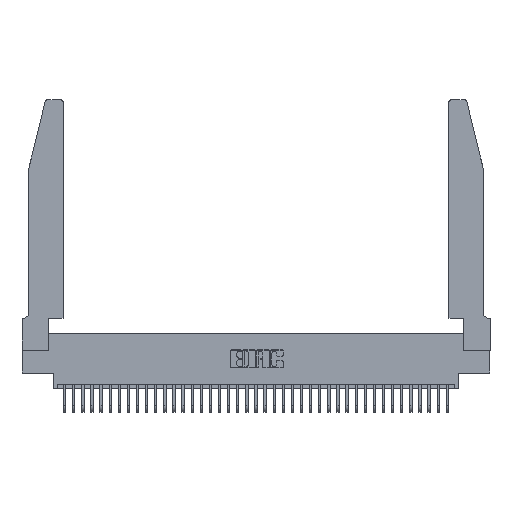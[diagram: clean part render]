
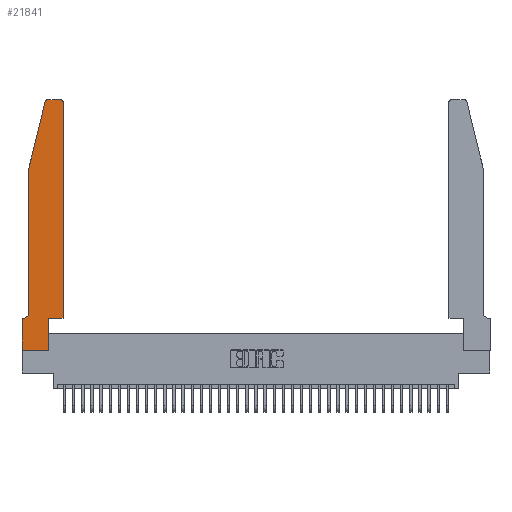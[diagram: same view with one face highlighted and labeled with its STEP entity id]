
A CAD part, top view. The second image highlights one B-rep face of the part: STEP entity #21841.
In plain terms, the highlighted planar face has unit normal (0, 0, 1).
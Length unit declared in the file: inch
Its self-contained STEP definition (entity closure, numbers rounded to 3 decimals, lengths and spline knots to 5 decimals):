
#62 = EDGE_CURVE ( 'NONE', #2987, #4222, #34412, .T. ) ;
#102 = VECTOR ( 'NONE', #3313, 39.37008 ) ;
#933 = VERTEX_POINT ( 'NONE', #10836 ) ;
#972 = CARTESIAN_POINT ( 'NONE',  ( 0., 0., 0.37 ) ) ;
#1541 = EDGE_CURVE ( 'NONE', #31274, #18560, #9662, .T. ) ;
#2202 = ORIENTED_EDGE ( 'NONE', *, *, #29389, .T. ) ;
#2729 = CARTESIAN_POINT ( 'NONE',  ( 0.4505, 0.35, 0.37 ) ) ;
#2750 = VERTEX_POINT ( 'NONE', #28711 ) ;
#2987 = VERTEX_POINT ( 'NONE', #12644 ) ;
#3313 = DIRECTION ( 'NONE',  ( 1., 0., 0. ) ) ;
#3594 = ORIENTED_EDGE ( 'NONE', *, *, #25880, .T. ) ;
#3938 = EDGE_CURVE ( 'NONE', #933, #15047, #12264, .T. ) ;
#4116 = ORIENTED_EDGE ( 'NONE', *, *, #21458, .T. ) ;
#4222 = VERTEX_POINT ( 'NONE', #32093 ) ;
#4388 = DIRECTION ( 'NONE',  ( 0., 0., -1. ) ) ;
#6137 = LINE ( 'NONE', #28819, #35675 ) ;
#6713 = DIRECTION ( 'NONE',  ( 0., 1., 0. ) ) ;
#6797 = CARTESIAN_POINT ( 'NONE',  ( 0.0755, 0.42, 0.37 ) ) ;
#7261 = AXIS2_PLACEMENT_3D ( 'NONE', #25074, #7840, #27955 ) ;
#7658 = ORIENTED_EDGE ( 'NONE', *, *, #17595, .T. ) ;
#7794 = CIRCLE ( 'NONE', #7261, 0.03 ) ;
#7840 = DIRECTION ( 'NONE',  ( 0., 0., 1. ) ) ;
#8736 = EDGE_LOOP ( 'NONE', ( #4116, #7658, #26403, #24208, #19255, #18488, #2202, #29838, #17821, #16942, #3594, #21818 ) ) ;
#9355 = LINE ( 'NONE', #22764, #23757 ) ;
#9662 = LINE ( 'NONE', #2729, #33421 ) ;
#10003 = DIRECTION ( 'NONE',  ( 0., 0., 1. ) ) ;
#10808 = DIRECTION ( 'NONE',  ( -1., 0., 0. ) ) ;
#10836 = CARTESIAN_POINT ( 'NONE',  ( 0.0055, 0.35, 0.37 ) ) ;
#11283 = VERTEX_POINT ( 'NONE', #972 ) ;
#11332 = CARTESIAN_POINT ( 'NONE',  ( 0.25487, 2.72718, 0.37 ) ) ;
#11401 = AXIS2_PLACEMENT_3D ( 'NONE', #27223, #10003, #30077 ) ;
#12264 = LINE ( 'NONE', #36436, #18083 ) ;
#12644 = CARTESIAN_POINT ( 'NONE',  ( 0.4505, 2.72, 0.37 ) ) ;
#12943 = LINE ( 'NONE', #35268, #28207 ) ;
#13743 = PLANE ( 'NONE',  #33267 ) ;
#13778 = CARTESIAN_POINT ( 'NONE',  ( 0.2865, 0., 0.37 ) ) ;
#14523 = DIRECTION ( 'NONE',  ( -1., 0., 0. ) ) ;
#15047 = VERTEX_POINT ( 'NONE', #26535 ) ;
#16609 = DIRECTION ( 'NONE',  ( 1., 0., 0. ) ) ;
#16890 = CARTESIAN_POINT ( 'NONE',  ( 0.0755, 2., 0.37 ) ) ;
#16942 = ORIENTED_EDGE ( 'NONE', *, *, #1541, .T. ) ;
#17369 = EDGE_CURVE ( 'NONE', #35594, #31274, #31142, .T. ) ;
#17595 = EDGE_CURVE ( 'NONE', #28158, #18311, #7794, .T. ) ;
#17821 = ORIENTED_EDGE ( 'NONE', *, *, #17369, .T. ) ;
#17947 = CARTESIAN_POINT ( 'NONE',  ( 0.4505, 0.35, 0.37 ) ) ;
#18083 = VECTOR ( 'NONE', #10808, 39.37008 ) ;
#18183 = DIRECTION ( 'NONE',  ( -0.239, -0.971, 0. ) ) ;
#18311 = VERTEX_POINT ( 'NONE', #11332 ) ;
#18488 = ORIENTED_EDGE ( 'NONE', *, *, #3938, .T. ) ;
#18560 = VERTEX_POINT ( 'NONE', #32467 ) ;
#19045 = CARTESIAN_POINT ( 'NONE',  ( 0.2865, 0.35, 0.37 ) ) ;
#19103 = VECTOR ( 'NONE', #29465, 39.37008 ) ;
#19255 = ORIENTED_EDGE ( 'NONE', *, *, #27281, .T. ) ;
#19598 = EDGE_CURVE ( 'NONE', #2750, #34151, #30082, .T. ) ;
#19892 = DIRECTION ( 'NONE',  ( 0., -1., 0. ) ) ;
#20191 = CARTESIAN_POINT ( 'NONE',  ( 0.284, 2.75, 0.37 ) ) ;
#20580 = CARTESIAN_POINT ( 'NONE',  ( 0., 0., 0.37 ) ) ;
#21005 = EDGE_CURVE ( 'NONE', #18311, #2750, #12943, .T. ) ;
#21458 = EDGE_CURVE ( 'NONE', #4222, #28158, #6137, .T. ) ;
#21643 = CARTESIAN_POINT ( 'NONE',  ( 0.0055, 0.42, 0.37 ) ) ;
#21818 = ORIENTED_EDGE ( 'NONE', *, *, #62, .T. ) ;
#21841 = ADVANCED_FACE ( 'NONE', ( #30803 ), #13743, .T. ) ;
#22279 = CARTESIAN_POINT ( 'NONE',  ( 0., 0.35, 0.37 ) ) ;
#22476 = VECTOR ( 'NONE', #34125, 39.37008 ) ;
#22714 = EDGE_CURVE ( 'NONE', #11283, #35594, #23139, .T. ) ;
#22764 = CARTESIAN_POINT ( 'NONE',  ( 0., 0., 0.37 ) ) ;
#22862 = DIRECTION ( 'NONE',  ( 1., 0., 0. ) ) ;
#23139 = LINE ( 'NONE', #20580, #102 ) ;
#23757 = VECTOR ( 'NONE', #19892, 39.37008 ) ;
#24208 = ORIENTED_EDGE ( 'NONE', *, *, #19598, .T. ) ;
#24542 = DIRECTION ( 'NONE',  ( -1., 0., 0. ) ) ;
#25074 = CARTESIAN_POINT ( 'NONE',  ( 0.284, 2.72, 0.37 ) ) ;
#25880 = EDGE_CURVE ( 'NONE', #18560, #2987, #33381, .T. ) ;
#26403 = ORIENTED_EDGE ( 'NONE', *, *, #21005, .T. ) ;
#26535 = CARTESIAN_POINT ( 'NONE',  ( 0., 0.35, 0.37 ) ) ;
#27223 = CARTESIAN_POINT ( 'NONE',  ( 0.4205, 2.72, 0.37 ) ) ;
#27281 = EDGE_CURVE ( 'NONE', #34151, #933, #29733, .T. ) ;
#27955 = DIRECTION ( 'NONE',  ( 1., 0., 0. ) ) ;
#28158 = VERTEX_POINT ( 'NONE', #20191 ) ;
#28207 = VECTOR ( 'NONE', #18183, 39.37008 ) ;
#28711 = CARTESIAN_POINT ( 'NONE',  ( 0.0755, 2., 0.37 ) ) ;
#28819 = CARTESIAN_POINT ( 'NONE',  ( 0.2605, 2.75, 0.37 ) ) ;
#29389 = EDGE_CURVE ( 'NONE', #15047, #11283, #9355, .T. ) ;
#29465 = DIRECTION ( 'NONE',  ( 0., 1., 0. ) ) ;
#29733 = CIRCLE ( 'NONE', #31621, 0.07 ) ;
#29838 = ORIENTED_EDGE ( 'NONE', *, *, #22714, .T. ) ;
#30077 = DIRECTION ( 'NONE',  ( 1., 0., 0. ) ) ;
#30082 = LINE ( 'NONE', #16890, #22476 ) ;
#30255 = VECTOR ( 'NONE', #6713, 39.37008 ) ;
#30803 = FACE_OUTER_BOUND ( 'NONE', #8736, .T. ) ;
#31142 = LINE ( 'NONE', #35240, #30255 ) ;
#31274 = VERTEX_POINT ( 'NONE', #19045 ) ;
#31621 = AXIS2_PLACEMENT_3D ( 'NONE', #21643, #4388, #24542 ) ;
#32093 = CARTESIAN_POINT ( 'NONE',  ( 0.4205, 2.75, 0.37 ) ) ;
#32467 = CARTESIAN_POINT ( 'NONE',  ( 0.4505, 0.35, 0.37 ) ) ;
#33267 = AXIS2_PLACEMENT_3D ( 'NONE', #22279, #33738, #16609 ) ;
#33381 = LINE ( 'NONE', #17947, #19103 ) ;
#33421 = VECTOR ( 'NONE', #22862, 39.37008 ) ;
#33738 = DIRECTION ( 'NONE',  ( 0., 0., 1. ) ) ;
#34125 = DIRECTION ( 'NONE',  ( 0., -1., 0. ) ) ;
#34151 = VERTEX_POINT ( 'NONE', #6797 ) ;
#34412 = CIRCLE ( 'NONE', #11401, 0.03 ) ;
#35240 = CARTESIAN_POINT ( 'NONE',  ( 0.2865, 0.35, 0.37 ) ) ;
#35268 = CARTESIAN_POINT ( 'NONE',  ( 0.0755, 2., 0.37 ) ) ;
#35594 = VERTEX_POINT ( 'NONE', #13778 ) ;
#35675 = VECTOR ( 'NONE', #14523, 39.37008 ) ;
#36436 = CARTESIAN_POINT ( 'NONE',  ( 0.0755, 0.35, 0.37 ) ) ;
